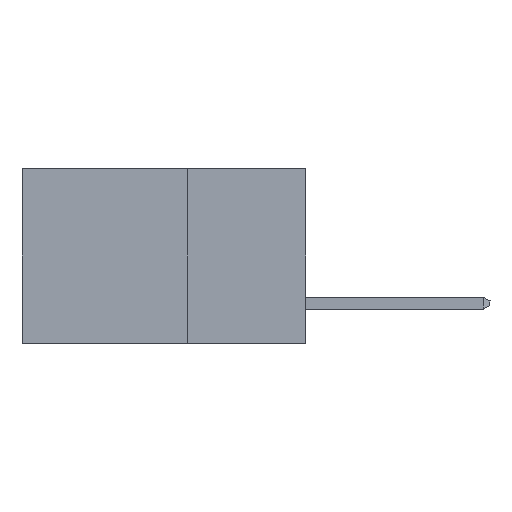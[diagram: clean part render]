
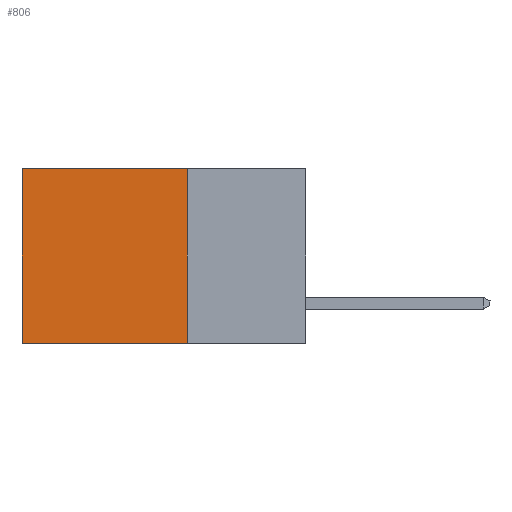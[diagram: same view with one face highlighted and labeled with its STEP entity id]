
A CAD part, left-side view. The second image highlights one B-rep face of the part: STEP entity #806.
In plain terms, the highlighted planar face has unit normal (-1, 0, 0).
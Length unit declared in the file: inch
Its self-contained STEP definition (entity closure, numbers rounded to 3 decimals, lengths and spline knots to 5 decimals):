
#254 = CARTESIAN_POINT ( 'NONE',  ( 0.298, 0.25, 0. ) ) ;
#710 = CARTESIAN_POINT ( 'NONE',  ( 0.298, 0.25, 0. ) ) ;
#806 = ADVANCED_FACE ( 'NONE', ( #9981 ), #13082, .F. ) ;
#1323 = LINE ( 'NONE', #710, #12439 ) ;
#1579 = CARTESIAN_POINT ( 'NONE',  ( 0.298, 0.6, 0. ) ) ;
#3010 = CARTESIAN_POINT ( 'NONE',  ( 0.298, 0.25, 0. ) ) ;
#3431 = ORIENTED_EDGE ( 'NONE', *, *, #15268, .T. ) ;
#3619 = VERTEX_POINT ( 'NONE', #3010 ) ;
#4884 = LINE ( 'NONE', #16314, #16044 ) ;
#5122 = VECTOR ( 'NONE', #15395, 39.37008 ) ;
#5670 = VERTEX_POINT ( 'NONE', #1579 ) ;
#6808 = DIRECTION ( 'NONE',  ( 1., 0., 0. ) ) ;
#7503 = VERTEX_POINT ( 'NONE', #7926 ) ;
#7926 = CARTESIAN_POINT ( 'NONE',  ( 0.298, 0.25, -0.37 ) ) ;
#9010 = VECTOR ( 'NONE', #13196, 39.37008 ) ;
#9402 = VERTEX_POINT ( 'NONE', #10043 ) ;
#9408 = CARTESIAN_POINT ( 'NONE',  ( 0.298, 0.6, 0. ) ) ;
#9981 = FACE_OUTER_BOUND ( 'NONE', #11506, .T. ) ;
#9998 = EDGE_CURVE ( 'NONE', #7503, #9402, #4884, .T. ) ;
#10043 = CARTESIAN_POINT ( 'NONE',  ( 0.298, 0.6, -0.37 ) ) ;
#10200 = ORIENTED_EDGE ( 'NONE', *, *, #12989, .T. ) ;
#10725 = DIRECTION ( 'NONE',  ( 0., 0., -1. ) ) ;
#11506 = EDGE_LOOP ( 'NONE', ( #10200, #12102, #14454, #3431 ) ) ;
#12102 = ORIENTED_EDGE ( 'NONE', *, *, #9998, .F. ) ;
#12439 = VECTOR ( 'NONE', #10725, 39.37008 ) ;
#12734 = LINE ( 'NONE', #9408, #9010 ) ;
#12989 = EDGE_CURVE ( 'NONE', #5670, #9402, #12734, .T. ) ;
#13082 = PLANE ( 'NONE',  #15033 ) ;
#13196 = DIRECTION ( 'NONE',  ( 0., 0., -1. ) ) ;
#14078 = LINE ( 'NONE', #254, #5122 ) ;
#14366 = CARTESIAN_POINT ( 'NONE',  ( 0.298, 0.25, 0. ) ) ;
#14454 = ORIENTED_EDGE ( 'NONE', *, *, #16337, .F. ) ;
#15017 = DIRECTION ( 'NONE',  ( 0., 1., 0. ) ) ;
#15033 = AXIS2_PLACEMENT_3D ( 'NONE', #14366, #6808, #15720 ) ;
#15268 = EDGE_CURVE ( 'NONE', #3619, #5670, #14078, .T. ) ;
#15395 = DIRECTION ( 'NONE',  ( 0., 1., 0. ) ) ;
#15720 = DIRECTION ( 'NONE',  ( 0., 0., -1. ) ) ;
#16044 = VECTOR ( 'NONE', #15017, 39.37008 ) ;
#16314 = CARTESIAN_POINT ( 'NONE',  ( 0.298, 0.25, -0.37 ) ) ;
#16337 = EDGE_CURVE ( 'NONE', #3619, #7503, #1323, .T. ) ;
